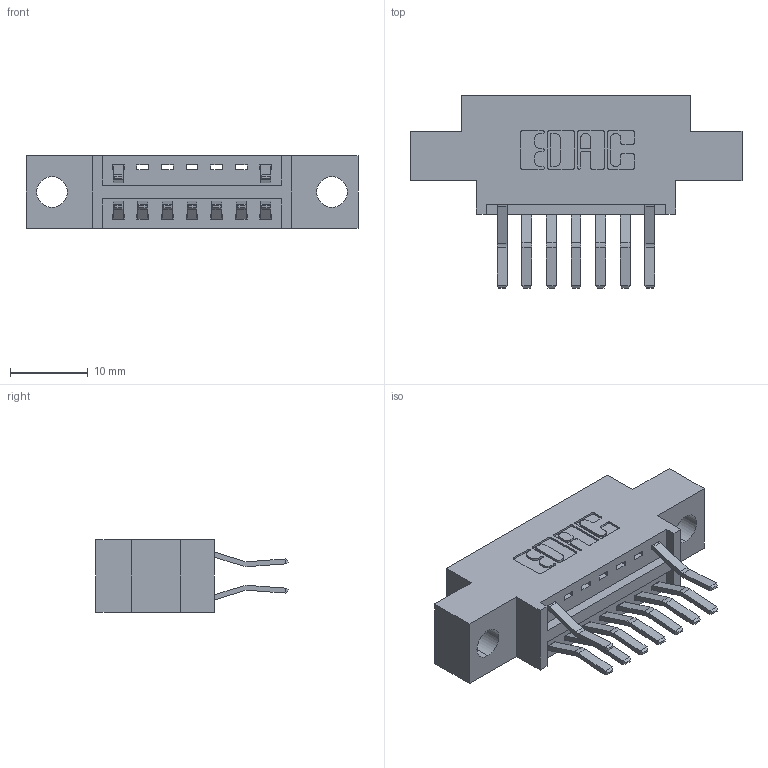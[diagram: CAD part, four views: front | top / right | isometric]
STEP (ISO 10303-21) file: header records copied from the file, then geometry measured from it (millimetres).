
FILE_DESCRIPTION (( 'STEP AP203' ), '1' );
FILE_NAME ('346-014-560-804.STEP', '2018-08-20T02:17:01', ( '' ), ( '' ), 'SwSTEP 2.0', 'SolidWorks 2016', '' );
FILE_SCHEMA (( 'CONFIG_CONTROL_DESIGN' ));
Length unit declared in the file: inch
Products named in the file (3): 346 Part_0.170 Offset - 0.156 Dia-TH; 345-292-001_560 Tail; 346-014-560-804
Assembly tree (10 placements, depth 2):
  346-014-560-804
    346 Part_0.170 Offset - 0.156 Dia-TH
    345-292-001_560 Tail  x9
Bounding box: 42.8 x 24.78 x 9.4 mm (x, y, z)
Volume: 3673.1 mm3; surface area: 4389.7 mm2
Topology: 10 solids, 10 shells, 642 faces, 1895 edges, 1250 vertices
Faces by surface type: plane 420, cylinder 222
Entity records: 9343 total; most frequent: CARTESIAN_POINT 1611, ORIENTED_EDGE 1550, DIRECTION 1469, EDGE_CURVE 775, LINE 611, VECTOR 611, VERTEX_POINT 514, AXIS2_PLACEMENT_3D 429
